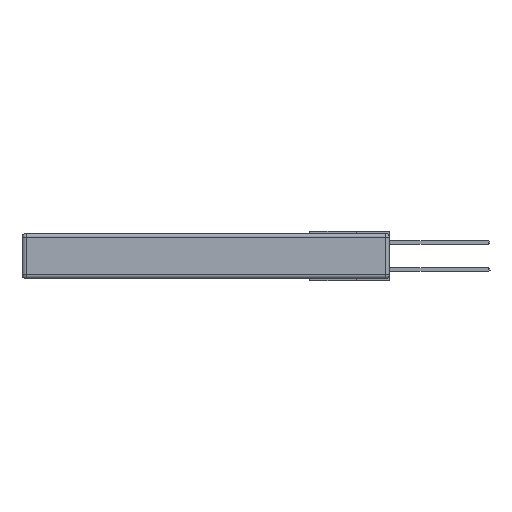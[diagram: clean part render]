
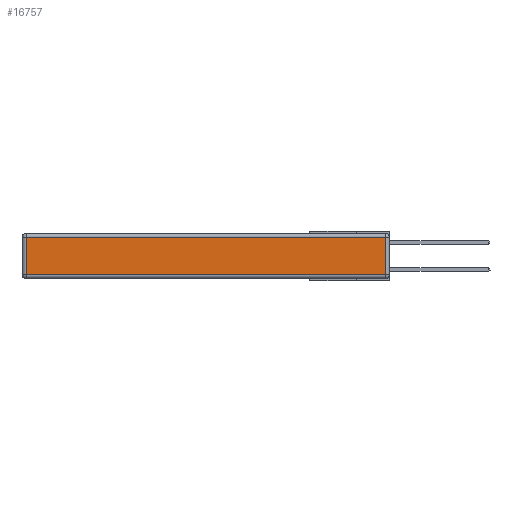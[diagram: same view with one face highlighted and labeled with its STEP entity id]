
A CAD part, left-side view. The second image highlights one B-rep face of the part: STEP entity #16757.
In plain terms, the highlighted planar face has unit normal (-1, 0, 0).
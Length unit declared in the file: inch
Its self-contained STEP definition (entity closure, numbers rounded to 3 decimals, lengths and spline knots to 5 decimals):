
#251 = DIRECTION ( 'NONE',  ( 0., 1., 0. ) ) ;
#1016 = VERTEX_POINT ( 'NONE', #6577 ) ;
#1017 = CARTESIAN_POINT ( 'NONE',  ( 0., 0.03, -0.03 ) ) ;
#1056 = ORIENTED_EDGE ( 'NONE', *, *, #1582, .T. ) ;
#1455 = CARTESIAN_POINT ( 'NONE',  ( 0., 2.72, -0.03 ) ) ;
#1582 = EDGE_CURVE ( 'NONE', #11225, #8301, #2127, .T. ) ;
#2127 = LINE ( 'NONE', #8527, #15783 ) ;
#3073 = VECTOR ( 'NONE', #15634, 39.37008 ) ;
#3589 = CARTESIAN_POINT ( 'NONE',  ( 0., 0., -0.343 ) ) ;
#3931 = ORIENTED_EDGE ( 'NONE', *, *, #13905, .T. ) ;
#4289 = DIRECTION ( 'NONE',  ( 0., 0., 1. ) ) ;
#4587 = LINE ( 'NONE', #5930, #3073 ) ;
#4617 = DIRECTION ( 'NONE',  ( 0., 0., 1. ) ) ;
#5230 = VECTOR ( 'NONE', #14533, 39.37008 ) ;
#5930 = CARTESIAN_POINT ( 'NONE',  ( 0., 0., -0.313 ) ) ;
#6121 = LINE ( 'NONE', #6158, #5230 ) ;
#6158 = CARTESIAN_POINT ( 'NONE',  ( 0., 2.72, -0.343 ) ) ;
#6577 = CARTESIAN_POINT ( 'NONE',  ( 0., 2.72, -0.313 ) ) ;
#8301 = VERTEX_POINT ( 'NONE', #1455 ) ;
#8358 = AXIS2_PLACEMENT_3D ( 'NONE', #3589, #16082, #4617 ) ;
#8475 = LINE ( 'NONE', #8555, #10871 ) ;
#8527 = CARTESIAN_POINT ( 'NONE',  ( 0., 2.75, -0.03 ) ) ;
#8555 = CARTESIAN_POINT ( 'NONE',  ( 0., 0.03, -0.343 ) ) ;
#9798 = EDGE_CURVE ( 'NONE', #8301, #1016, #6121, .T. ) ;
#10119 = VERTEX_POINT ( 'NONE', #10930 ) ;
#10871 = VECTOR ( 'NONE', #4289, 39.37008 ) ;
#10930 = CARTESIAN_POINT ( 'NONE',  ( 0., 0.03, -0.313 ) ) ;
#11225 = VERTEX_POINT ( 'NONE', #1017 ) ;
#11962 = EDGE_LOOP ( 'NONE', ( #13435, #3931, #1056, #14582 ) ) ;
#13435 = ORIENTED_EDGE ( 'NONE', *, *, #17918, .T. ) ;
#13905 = EDGE_CURVE ( 'NONE', #10119, #11225, #8475, .T. ) ;
#14533 = DIRECTION ( 'NONE',  ( 0., 0., -1. ) ) ;
#14582 = ORIENTED_EDGE ( 'NONE', *, *, #9798, .T. ) ;
#15544 = FACE_OUTER_BOUND ( 'NONE', #11962, .T. ) ;
#15634 = DIRECTION ( 'NONE',  ( 0., -1., 0. ) ) ;
#15783 = VECTOR ( 'NONE', #251, 39.37008 ) ;
#16082 = DIRECTION ( 'NONE',  ( -1., 0., 0. ) ) ;
#16757 = ADVANCED_FACE ( 'NONE', ( #15544 ), #17581, .T. ) ;
#17581 = PLANE ( 'NONE',  #8358 ) ;
#17918 = EDGE_CURVE ( 'NONE', #1016, #10119, #4587, .T. ) ;
